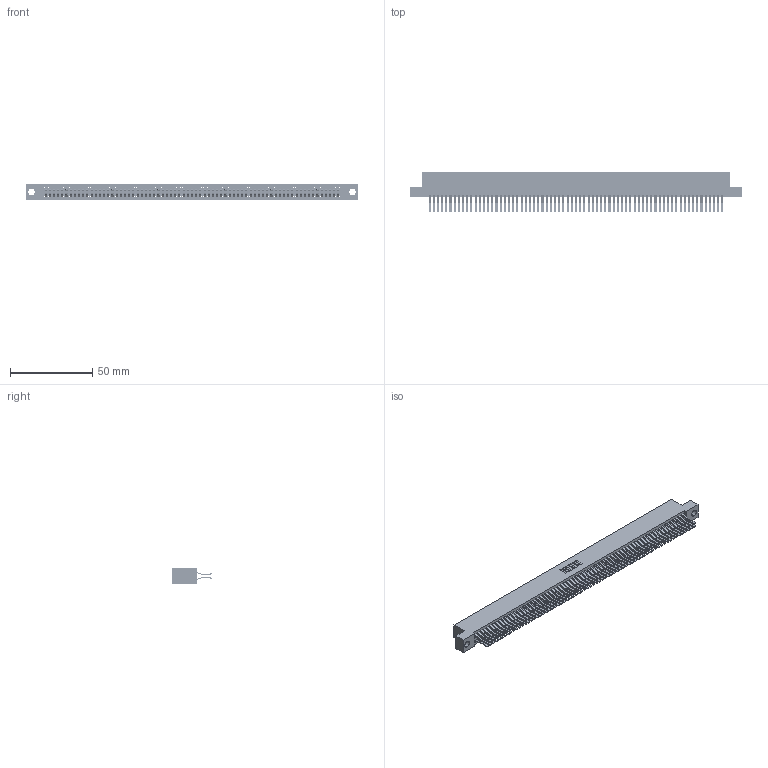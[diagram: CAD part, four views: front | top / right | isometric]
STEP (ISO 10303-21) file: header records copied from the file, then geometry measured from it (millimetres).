
FILE_DESCRIPTION (( 'STEP AP203' ), '1' );
FILE_NAME ('395-142-560-204.STEP', '2018-12-06T05:23:54', ( '' ), ( '' ), 'SwSTEP 2.0', 'SolidWorks 2016', '' );
FILE_SCHEMA (( 'CONFIG_CONTROL_DESIGN' ));
Length unit declared in the file: inch
Products named in the file (3): 345-292-001_560 Tail; 345 Part_Flush Mounting Lugs - 0.156 Dia-TH; 395-142-560-204
Assembly tree (143 placements, depth 2):
  395-142-560-204
    345 Part_Flush Mounting Lugs - 0.156 Dia-TH
    345-292-001_560 Tail  x142
Bounding box: 201.55 x 24.45 x 9.4 mm (x, y, z)
Volume: 20690.8 mm3; surface area: 33355.1 mm2
Topology: 143 solids, 143 shells, 7510 faces, 22351 edges, 14710 vertices
Faces by surface type: plane 4766, cylinder 2744
Entity records: 51895 total; most frequent: CARTESIAN_POINT 8672, ORIENTED_EDGE 8606, DIRECTION 7615, EDGE_CURVE 4303, LINE 3883, VECTOR 3883, VERTEX_POINT 2866, AXIS2_PLACEMENT_3D 1866
